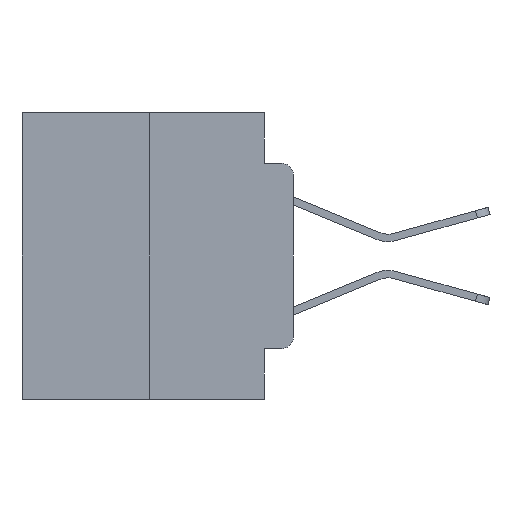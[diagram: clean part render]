
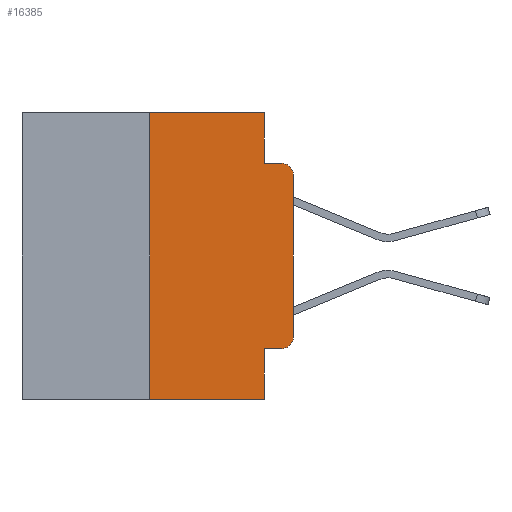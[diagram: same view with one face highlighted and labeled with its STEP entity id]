
A CAD part, left-side view. The second image highlights one B-rep face of the part: STEP entity #16385.
In plain terms, the highlighted planar face has unit normal (-1, 0, 0).
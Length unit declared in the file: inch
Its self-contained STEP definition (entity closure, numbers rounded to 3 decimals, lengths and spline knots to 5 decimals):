
#153 = ORIENTED_EDGE ( 'NONE', *, *, #12737, .T. ) ;
#478 = CARTESIAN_POINT ( 'NONE',  ( 0., 0.051, -0.5 ) ) ;
#766 = DIRECTION ( 'NONE',  ( -1., 0., 0. ) ) ;
#910 = DIRECTION ( 'NONE',  ( 0., 0., 1. ) ) ;
#1206 = VERTEX_POINT ( 'NONE', #3051 ) ;
#1343 = DIRECTION ( 'NONE',  ( 0., -1., 0. ) ) ;
#1520 = VERTEX_POINT ( 'NONE', #26741 ) ;
#1646 = VERTEX_POINT ( 'NONE', #12743 ) ;
#1691 = LINE ( 'NONE', #25610, #20716 ) ;
#2134 = CIRCLE ( 'NONE', #16075, 0.02 ) ;
#2756 = CIRCLE ( 'NONE', #16345, 0.02 ) ;
#3051 = CARTESIAN_POINT ( 'NONE',  ( 0., 0., -0.1085 ) ) ;
#3396 = ORIENTED_EDGE ( 'NONE', *, *, #18351, .F. ) ;
#3928 = EDGE_CURVE ( 'NONE', #17564, #14480, #9906, .T. ) ;
#4014 = ORIENTED_EDGE ( 'NONE', *, *, #22433, .F. ) ;
#4148 = CARTESIAN_POINT ( 'NONE',  ( 0., 0.051, 0. ) ) ;
#4172 = DIRECTION ( 'NONE',  ( 0., 0., -1. ) ) ;
#4673 = ORIENTED_EDGE ( 'NONE', *, *, #3928, .T. ) ;
#4821 = VECTOR ( 'NONE', #13722, 39.37008 ) ;
#5142 = LINE ( 'NONE', #13544, #4821 ) ;
#5166 = EDGE_CURVE ( 'NONE', #1520, #24703, #1691, .T. ) ;
#6193 = VERTEX_POINT ( 'NONE', #19973 ) ;
#6387 = CARTESIAN_POINT ( 'NONE',  ( 0., 0.25, -0.5 ) ) ;
#7087 = CARTESIAN_POINT ( 'NONE',  ( 0., 0.051, -0.4115 ) ) ;
#7243 = CARTESIAN_POINT ( 'NONE',  ( 0., 0.473, 0. ) ) ;
#8214 = DIRECTION ( 'NONE',  ( 0., 0., -1. ) ) ;
#8241 = EDGE_LOOP ( 'NONE', ( #153, #10093, #4014, #17746, #13591, #14153, #17492, #3396, #4673, #24706 ) ) ;
#9280 = DIRECTION ( 'NONE',  ( 0., -1., 0. ) ) ;
#9906 = LINE ( 'NONE', #25138, #10821 ) ;
#9934 = EDGE_CURVE ( 'NONE', #24703, #6193, #26493, .T. ) ;
#10065 = CARTESIAN_POINT ( 'NONE',  ( 0., 0., -0.3915 ) ) ;
#10093 = ORIENTED_EDGE ( 'NONE', *, *, #21607, .T. ) ;
#10116 = FACE_OUTER_BOUND ( 'NONE', #8241, .T. ) ;
#10821 = VECTOR ( 'NONE', #25044, 39.37008 ) ;
#10948 = VECTOR ( 'NONE', #1343, 39.37008 ) ;
#11141 = VERTEX_POINT ( 'NONE', #6387 ) ;
#12182 = LINE ( 'NONE', #13275, #23439 ) ;
#12404 = CARTESIAN_POINT ( 'NONE',  ( 0., 0.02, -0.1085 ) ) ;
#12737 = EDGE_CURVE ( 'NONE', #17928, #1206, #12182, .T. ) ;
#12743 = CARTESIAN_POINT ( 'NONE',  ( 0., 0.02, -0.0885 ) ) ;
#13142 = CARTESIAN_POINT ( 'NONE',  ( 0., 0.02, -0.3915 ) ) ;
#13219 = CARTESIAN_POINT ( 'NONE',  ( 0., 0.051, -0.0885 ) ) ;
#13275 = CARTESIAN_POINT ( 'NONE',  ( 0., 0., 0. ) ) ;
#13498 = DIRECTION ( 'NONE',  ( 0., -1., 0. ) ) ;
#13544 = CARTESIAN_POINT ( 'NONE',  ( 0., 0.051, 0. ) ) ;
#13591 = ORIENTED_EDGE ( 'NONE', *, *, #5166, .F. ) ;
#13722 = DIRECTION ( 'NONE',  ( 0., 0., -1. ) ) ;
#13890 = VECTOR ( 'NONE', #8214, 39.37008 ) ;
#13910 = VECTOR ( 'NONE', #9280, 39.37008 ) ;
#14153 = ORIENTED_EDGE ( 'NONE', *, *, #14756, .F. ) ;
#14480 = VERTEX_POINT ( 'NONE', #16754 ) ;
#14552 = LINE ( 'NONE', #13219, #13910 ) ;
#14756 = EDGE_CURVE ( 'NONE', #11141, #1520, #21404, .T. ) ;
#15195 = DIRECTION ( 'NONE',  ( 0., 0., -1. ) ) ;
#15451 = DIRECTION ( 'NONE',  ( 0., 0., -1. ) ) ;
#15499 = DIRECTION ( 'NONE',  ( 0., 0., 1. ) ) ;
#16075 = AXIS2_PLACEMENT_3D ( 'NONE', #13142, #766, #15195 ) ;
#16184 = DIRECTION ( 'NONE',  ( -1., 0., 0. ) ) ;
#16345 = AXIS2_PLACEMENT_3D ( 'NONE', #12404, #16184, #4172 ) ;
#16385 = ADVANCED_FACE ( 'NONE', ( #10116 ), #17339, .F. ) ;
#16754 = CARTESIAN_POINT ( 'NONE',  ( 0., 0.02, -0.4115 ) ) ;
#17339 = PLANE ( 'NONE',  #20233 ) ;
#17492 = ORIENTED_EDGE ( 'NONE', *, *, #18409, .T. ) ;
#17532 = VECTOR ( 'NONE', #15499, 39.37008 ) ;
#17564 = VERTEX_POINT ( 'NONE', #7087 ) ;
#17746 = ORIENTED_EDGE ( 'NONE', *, *, #9934, .F. ) ;
#17928 = VERTEX_POINT ( 'NONE', #10065 ) ;
#18049 = LINE ( 'NONE', #26094, #10948 ) ;
#18351 = EDGE_CURVE ( 'NONE', #17564, #24221, #5142, .T. ) ;
#18409 = EDGE_CURVE ( 'NONE', #11141, #24221, #18049, .T. ) ;
#19374 = CARTESIAN_POINT ( 'NONE',  ( 0., 0.25, 0. ) ) ;
#19412 = DIRECTION ( 'NONE',  ( 1., 0., 0. ) ) ;
#19973 = CARTESIAN_POINT ( 'NONE',  ( 0., 0.051, -0.0885 ) ) ;
#20233 = AXIS2_PLACEMENT_3D ( 'NONE', #7243, #19412, #15451 ) ;
#20716 = VECTOR ( 'NONE', #13498, 39.37008 ) ;
#21404 = LINE ( 'NONE', #19374, #17532 ) ;
#21607 = EDGE_CURVE ( 'NONE', #1206, #1646, #2756, .T. ) ;
#22433 = EDGE_CURVE ( 'NONE', #6193, #1646, #14552, .T. ) ;
#23439 = VECTOR ( 'NONE', #910, 39.37008 ) ;
#24221 = VERTEX_POINT ( 'NONE', #478 ) ;
#24703 = VERTEX_POINT ( 'NONE', #4148 ) ;
#24706 = ORIENTED_EDGE ( 'NONE', *, *, #25152, .T. ) ;
#24793 = CARTESIAN_POINT ( 'NONE',  ( 0., 0.051, 0. ) ) ;
#25044 = DIRECTION ( 'NONE',  ( 0., -1., 0. ) ) ;
#25138 = CARTESIAN_POINT ( 'NONE',  ( 0., 0.051, -0.4115 ) ) ;
#25152 = EDGE_CURVE ( 'NONE', #14480, #17928, #2134, .T. ) ;
#25610 = CARTESIAN_POINT ( 'NONE',  ( 0., 0.473, 0. ) ) ;
#26094 = CARTESIAN_POINT ( 'NONE',  ( 0., 0.473, -0.5 ) ) ;
#26493 = LINE ( 'NONE', #24793, #13890 ) ;
#26741 = CARTESIAN_POINT ( 'NONE',  ( 0., 0.25, 0. ) ) ;
